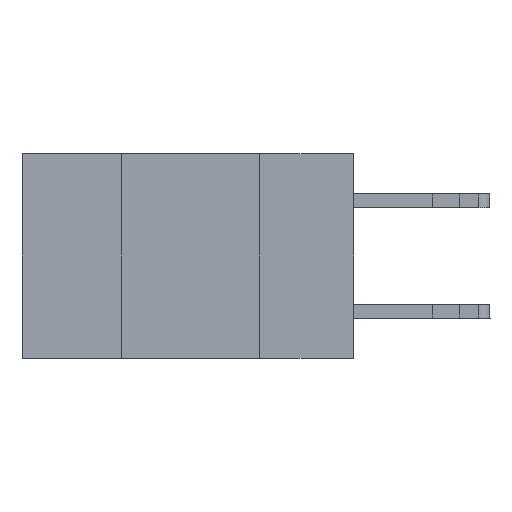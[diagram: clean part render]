
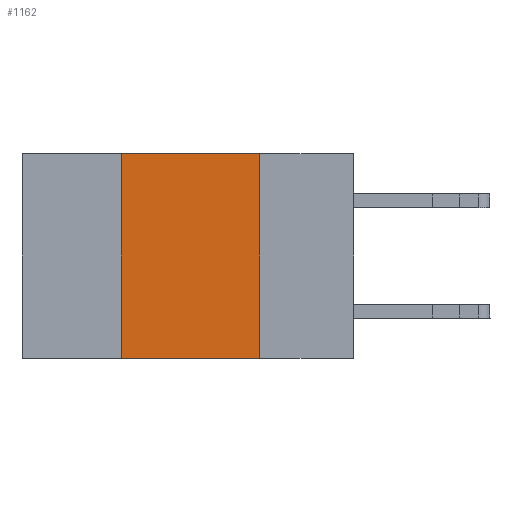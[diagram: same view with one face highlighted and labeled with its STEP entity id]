
A CAD part, left-side view. The second image highlights one B-rep face of the part: STEP entity #1162.
In plain terms, the highlighted planar face has unit normal (-1, 0, 0).
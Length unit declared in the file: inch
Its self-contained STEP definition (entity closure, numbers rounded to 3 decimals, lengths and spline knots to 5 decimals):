
#30 = LINE ( 'NONE', #13069, #12917 ) ;
#519 = VERTEX_POINT ( 'NONE', #11009 ) ;
#597 = DIRECTION ( 'NONE',  ( 0., 0., -1. ) ) ;
#754 = CARTESIAN_POINT ( 'NONE',  ( 0., 0.42, 0. ) ) ;
#969 = VECTOR ( 'NONE', #15374, 39.37008 ) ;
#1162 = ADVANCED_FACE ( 'NONE', ( #14870 ), #2951, .F. ) ;
#2129 = DIRECTION ( 'NONE',  ( 0., -1., 0. ) ) ;
#2457 = EDGE_LOOP ( 'NONE', ( #4181, #6942, #13373, #5815 ) ) ;
#2875 = EDGE_CURVE ( 'NONE', #11597, #5580, #2933, .T. ) ;
#2933 = LINE ( 'NONE', #7893, #8296 ) ;
#2951 = PLANE ( 'NONE',  #3715 ) ;
#3215 = CARTESIAN_POINT ( 'NONE',  ( 0., 0.6, 0. ) ) ;
#3327 = DIRECTION ( 'NONE',  ( 0., 0., 1. ) ) ;
#3715 = AXIS2_PLACEMENT_3D ( 'NONE', #15031, #7757, #597 ) ;
#4181 = ORIENTED_EDGE ( 'NONE', *, *, #2875, .F. ) ;
#4261 = EDGE_CURVE ( 'NONE', #519, #5580, #30, .T. ) ;
#5580 = VERTEX_POINT ( 'NONE', #5930 ) ;
#5815 = ORIENTED_EDGE ( 'NONE', *, *, #4261, .T. ) ;
#5930 = CARTESIAN_POINT ( 'NONE',  ( 0., 0.17, -0.37 ) ) ;
#6942 = ORIENTED_EDGE ( 'NONE', *, *, #11416, .F. ) ;
#7331 = CARTESIAN_POINT ( 'NONE',  ( 0., 0.42, 0. ) ) ;
#7757 = DIRECTION ( 'NONE',  ( 1., 0., 0. ) ) ;
#7893 = CARTESIAN_POINT ( 'NONE',  ( 0., 0.17, 0. ) ) ;
#8296 = VECTOR ( 'NONE', #11432, 39.37008 ) ;
#10825 = VECTOR ( 'NONE', #3327, 39.37008 ) ;
#10951 = VERTEX_POINT ( 'NONE', #754 ) ;
#11009 = CARTESIAN_POINT ( 'NONE',  ( 0., 0.42, -0.37 ) ) ;
#11416 = EDGE_CURVE ( 'NONE', #10951, #11597, #13984, .T. ) ;
#11432 = DIRECTION ( 'NONE',  ( 0., 0., -1. ) ) ;
#11597 = VERTEX_POINT ( 'NONE', #14354 ) ;
#11676 = LINE ( 'NONE', #7331, #10825 ) ;
#12917 = VECTOR ( 'NONE', #2129, 39.37008 ) ;
#13069 = CARTESIAN_POINT ( 'NONE',  ( 0., 0.6, -0.37 ) ) ;
#13373 = ORIENTED_EDGE ( 'NONE', *, *, #14055, .F. ) ;
#13984 = LINE ( 'NONE', #3215, #969 ) ;
#14055 = EDGE_CURVE ( 'NONE', #519, #10951, #11676, .T. ) ;
#14354 = CARTESIAN_POINT ( 'NONE',  ( 0., 0.17, 0. ) ) ;
#14870 = FACE_OUTER_BOUND ( 'NONE', #2457, .T. ) ;
#15031 = CARTESIAN_POINT ( 'NONE',  ( 0., 0.6, 0. ) ) ;
#15374 = DIRECTION ( 'NONE',  ( 0., -1., 0. ) ) ;
